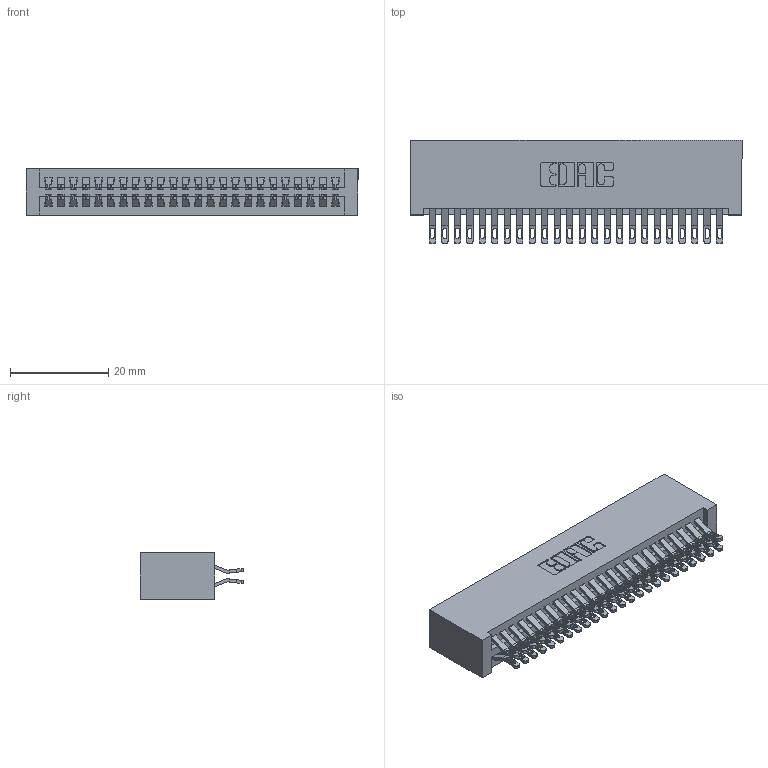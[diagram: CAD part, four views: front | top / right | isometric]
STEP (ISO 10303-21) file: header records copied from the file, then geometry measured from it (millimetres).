
FILE_DESCRIPTION (( 'STEP AP203' ), '1' );
FILE_NAME ('345-048-555-201.STEP', '2019-10-29T05:20:40', ( '' ), ( '' ), 'SwSTEP 2.0', 'SolidWorks 2016', '' );
FILE_SCHEMA (( 'CONFIG_CONTROL_DESIGN' ));
Length unit declared in the file: inch
Products named in the file (3): 345-292-001_555 Tail; 345-048-555-201; 345 Part_No Mounting Lugs
Assembly tree (49 placements, depth 2):
  345-048-555-201
    345 Part_No Mounting Lugs
    345-292-001_555 Tail  x48
Bounding box: 67.56 x 21.13 x 9.4 mm (x, y, z)
Volume: 7151.3 mm3; surface area: 11009.7 mm2
Topology: 49 solids, 49 shells, 2806 faces, 8813 edges, 5874 vertices
Faces by surface type: plane 1564, cylinder 1242
Entity records: 21303 total; most frequent: CARTESIAN_POINT 3622, ORIENTED_EDGE 3526, DIRECTION 3179, EDGE_CURVE 1763, LINE 1523, VECTOR 1523, VERTEX_POINT 1174, AXIS2_PLACEMENT_3D 828
